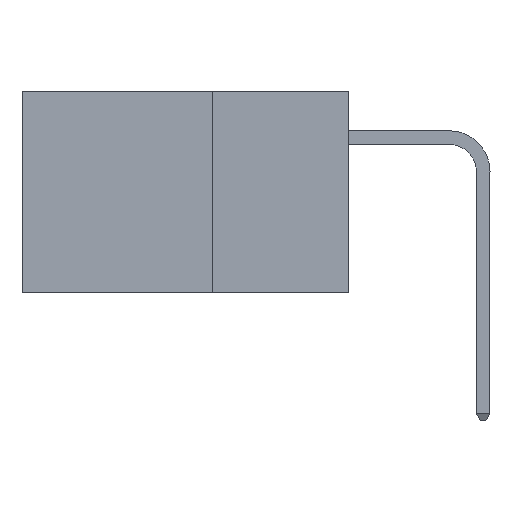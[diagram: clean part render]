
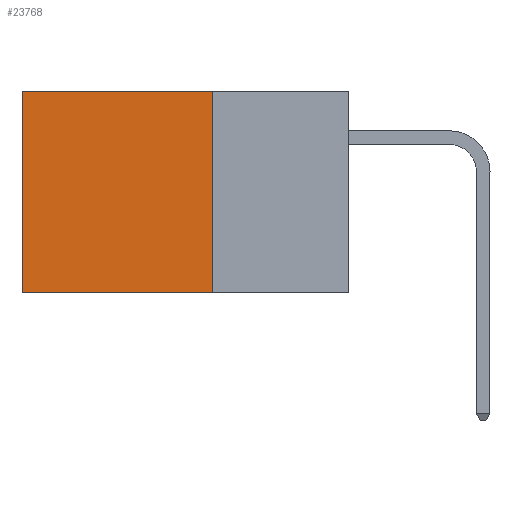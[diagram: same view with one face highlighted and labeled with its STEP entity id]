
A CAD part, left-side view. The second image highlights one B-rep face of the part: STEP entity #23768.
In plain terms, the highlighted planar face has unit normal (-1, 0, 0).
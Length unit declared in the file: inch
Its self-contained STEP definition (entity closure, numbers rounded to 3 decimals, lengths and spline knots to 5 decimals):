
#1058 = CARTESIAN_POINT ( 'NONE',  ( 0.2875, 0.6, -0.37 ) ) ;
#2783 = EDGE_CURVE ( 'NONE', #14613, #13936, #19313, .T. ) ;
#3688 = DIRECTION ( 'NONE',  ( 0., 0., -1. ) ) ;
#3766 = ORIENTED_EDGE ( 'NONE', *, *, #16932, .F. ) ;
#4863 = CARTESIAN_POINT ( 'NONE',  ( 0.2875, 0.6, 0. ) ) ;
#6311 = VECTOR ( 'NONE', #14698, 39.37008 ) ;
#8826 = CARTESIAN_POINT ( 'NONE',  ( 0.2875, 0.25, 0. ) ) ;
#9585 = VECTOR ( 'NONE', #3688, 39.37008 ) ;
#9976 = LINE ( 'NONE', #8826, #28328 ) ;
#10238 = LINE ( 'NONE', #18821, #17798 ) ;
#11174 = ORIENTED_EDGE ( 'NONE', *, *, #21559, .T. ) ;
#13284 = ORIENTED_EDGE ( 'NONE', *, *, #26369, .F. ) ;
#13936 = VERTEX_POINT ( 'NONE', #1058 ) ;
#14613 = VERTEX_POINT ( 'NONE', #22142 ) ;
#14698 = DIRECTION ( 'NONE',  ( 0., 1., 0. ) ) ;
#15548 = DIRECTION ( 'NONE',  ( 0., 0., -1. ) ) ;
#16932 = EDGE_CURVE ( 'NONE', #27531, #13936, #10238, .T. ) ;
#17798 = VECTOR ( 'NONE', #31026, 39.37008 ) ;
#18123 = PLANE ( 'NONE',  #19586 ) ;
#18493 = DIRECTION ( 'NONE',  ( 0., 0., -1. ) ) ;
#18821 = CARTESIAN_POINT ( 'NONE',  ( 0.2875, 0.25, -0.37 ) ) ;
#19313 = LINE ( 'NONE', #4863, #9585 ) ;
#19586 = AXIS2_PLACEMENT_3D ( 'NONE', #24875, #22881, #15548 ) ;
#21559 = EDGE_CURVE ( 'NONE', #28996, #14613, #30290, .T. ) ;
#21853 = CARTESIAN_POINT ( 'NONE',  ( 0.2875, 0.25, 0. ) ) ;
#22142 = CARTESIAN_POINT ( 'NONE',  ( 0.2875, 0.6, 0. ) ) ;
#22739 = CARTESIAN_POINT ( 'NONE',  ( 0.2875, 0.25, 0. ) ) ;
#22881 = DIRECTION ( 'NONE',  ( 1., 0., 0. ) ) ;
#23602 = ORIENTED_EDGE ( 'NONE', *, *, #2783, .T. ) ;
#23768 = ADVANCED_FACE ( 'NONE', ( #24318 ), #18123, .F. ) ;
#24318 = FACE_OUTER_BOUND ( 'NONE', #29592, .T. ) ;
#24875 = CARTESIAN_POINT ( 'NONE',  ( 0.2875, 0.25, 0. ) ) ;
#26369 = EDGE_CURVE ( 'NONE', #28996, #27531, #9976, .T. ) ;
#27531 = VERTEX_POINT ( 'NONE', #30517 ) ;
#28328 = VECTOR ( 'NONE', #18493, 39.37008 ) ;
#28996 = VERTEX_POINT ( 'NONE', #22739 ) ;
#29592 = EDGE_LOOP ( 'NONE', ( #23602, #3766, #13284, #11174 ) ) ;
#30290 = LINE ( 'NONE', #21853, #6311 ) ;
#30517 = CARTESIAN_POINT ( 'NONE',  ( 0.2875, 0.25, -0.37 ) ) ;
#31026 = DIRECTION ( 'NONE',  ( 0., 1., 0. ) ) ;
